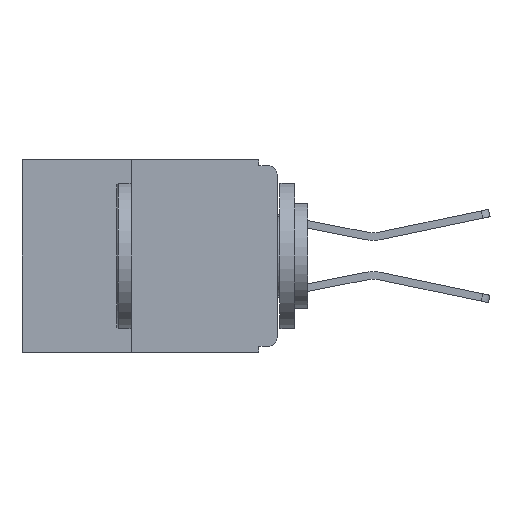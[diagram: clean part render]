
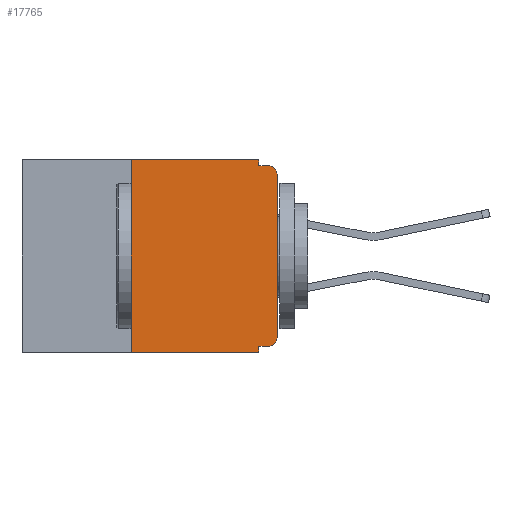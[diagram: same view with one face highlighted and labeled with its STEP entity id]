
A CAD part, left-side view. The second image highlights one B-rep face of the part: STEP entity #17765.
In plain terms, the highlighted planar face has unit normal (-1, 0, 0).
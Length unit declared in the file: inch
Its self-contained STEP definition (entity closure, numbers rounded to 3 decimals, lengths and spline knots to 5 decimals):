
#1190 = EDGE_CURVE ( 'NONE', #27178, #13181, #30315, .T. ) ;
#1698 = CARTESIAN_POINT ( 'NONE',  ( 0., 0.031, -0.32 ) ) ;
#1890 = ORIENTED_EDGE ( 'NONE', *, *, #15229, .T. ) ;
#2044 = CARTESIAN_POINT ( 'NONE',  ( 0., 0., -0.32 ) ) ;
#2105 = VERTEX_POINT ( 'NONE', #14401 ) ;
#2422 = FACE_OUTER_BOUND ( 'NONE', #13908, .T. ) ;
#2535 = EDGE_CURVE ( 'NONE', #2105, #15382, #26771, .T. ) ;
#3551 = DIRECTION ( 'NONE',  ( 0., -1., 0. ) ) ;
#4526 = VERTEX_POINT ( 'NONE', #29566 ) ;
#4619 = CIRCLE ( 'NONE', #5890, 0.015 ) ;
#4720 = DIRECTION ( 'NONE',  ( 0., 0., -1. ) ) ;
#4941 = ORIENTED_EDGE ( 'NONE', *, *, #5636, .F. ) ;
#5055 = EDGE_CURVE ( 'NONE', #17102, #7187, #18247, .T. ) ;
#5384 = CARTESIAN_POINT ( 'NONE',  ( 0., 0.015, -0.025 ) ) ;
#5439 = CARTESIAN_POINT ( 'NONE',  ( 0., 0.437, 0. ) ) ;
#5475 = CARTESIAN_POINT ( 'NONE',  ( 0., 0.031, 0. ) ) ;
#5487 = DIRECTION ( 'NONE',  ( 0., -1., 0. ) ) ;
#5618 = VECTOR ( 'NONE', #21946, 39.37008 ) ;
#5636 = EDGE_CURVE ( 'NONE', #7187, #4526, #25058, .T. ) ;
#5670 = VERTEX_POINT ( 'NONE', #21324 ) ;
#5890 = AXIS2_PLACEMENT_3D ( 'NONE', #5384, #22429, #7809 ) ;
#6074 = ORIENTED_EDGE ( 'NONE', *, *, #1190, .F. ) ;
#7187 = VERTEX_POINT ( 'NONE', #10266 ) ;
#7809 = DIRECTION ( 'NONE',  ( 0., 0., -1. ) ) ;
#8346 = CARTESIAN_POINT ( 'NONE',  ( 0., 0.015, -0.305 ) ) ;
#8969 = CARTESIAN_POINT ( 'NONE',  ( 0., 0.25, 0. ) ) ;
#9055 = CARTESIAN_POINT ( 'NONE',  ( 0., 0., 0. ) ) ;
#9332 = EDGE_CURVE ( 'NONE', #27122, #5670, #20014, .T. ) ;
#10266 = CARTESIAN_POINT ( 'NONE',  ( 0., 0.031, -0.01 ) ) ;
#10271 = CARTESIAN_POINT ( 'NONE',  ( 0., 0.437, -0.33 ) ) ;
#10335 = EDGE_CURVE ( 'NONE', #2105, #13181, #24128, .T. ) ;
#10840 = DIRECTION ( 'NONE',  ( 0., 0., -1. ) ) ;
#11438 = LINE ( 'NONE', #25497, #30891 ) ;
#11677 = VERTEX_POINT ( 'NONE', #17788 ) ;
#11937 = VECTOR ( 'NONE', #5487, 39.37008 ) ;
#12082 = CARTESIAN_POINT ( 'NONE',  ( 0., 0.031, 0. ) ) ;
#12587 = ORIENTED_EDGE ( 'NONE', *, *, #30724, .F. ) ;
#12804 = DIRECTION ( 'NONE',  ( 1., 0., 0. ) ) ;
#13092 = VECTOR ( 'NONE', #27851, 39.37008 ) ;
#13181 = VERTEX_POINT ( 'NONE', #20124 ) ;
#13642 = CARTESIAN_POINT ( 'NONE',  ( 0., 0., -0.305 ) ) ;
#13786 = EDGE_CURVE ( 'NONE', #5670, #4526, #4619, .T. ) ;
#13908 = EDGE_LOOP ( 'NONE', ( #14840, #23605, #4941, #25131, #19818, #14471, #29713, #6074, #12587, #1890 ) ) ;
#13986 = EDGE_CURVE ( 'NONE', #15382, #17102, #11438, .T. ) ;
#14401 = CARTESIAN_POINT ( 'NONE',  ( 0., 0.25, -0.33 ) ) ;
#14471 = ORIENTED_EDGE ( 'NONE', *, *, #2535, .F. ) ;
#14840 = ORIENTED_EDGE ( 'NONE', *, *, #9332, .T. ) ;
#15229 = EDGE_CURVE ( 'NONE', #11677, #27122, #18995, .T. ) ;
#15382 = VERTEX_POINT ( 'NONE', #8969 ) ;
#17102 = VERTEX_POINT ( 'NONE', #12082 ) ;
#17206 = CARTESIAN_POINT ( 'NONE',  ( 0., 0.031, -0.33 ) ) ;
#17574 = AXIS2_PLACEMENT_3D ( 'NONE', #8346, #25427, #10840 ) ;
#17765 = ADVANCED_FACE ( 'NONE', ( #2422 ), #27368, .F. ) ;
#17788 = CARTESIAN_POINT ( 'NONE',  ( 0., 0.015, -0.32 ) ) ;
#18247 = LINE ( 'NONE', #5475, #30434 ) ;
#18971 = DIRECTION ( 'NONE',  ( 0., 0., -1. ) ) ;
#18995 = CIRCLE ( 'NONE', #17574, 0.015 ) ;
#19093 = DIRECTION ( 'NONE',  ( 0., 1., 0. ) ) ;
#19818 = ORIENTED_EDGE ( 'NONE', *, *, #13986, .F. ) ;
#20014 = LINE ( 'NONE', #9055, #26473 ) ;
#20124 = CARTESIAN_POINT ( 'NONE',  ( 0., 0.031, -0.33 ) ) ;
#21324 = CARTESIAN_POINT ( 'NONE',  ( 0., 0., -0.025 ) ) ;
#21946 = DIRECTION ( 'NONE',  ( 0., -1., 0. ) ) ;
#22004 = VECTOR ( 'NONE', #19093, 39.37008 ) ;
#22165 = CARTESIAN_POINT ( 'NONE',  ( 0., 0., -0.01 ) ) ;
#22429 = DIRECTION ( 'NONE',  ( -1., 0., 0. ) ) ;
#23605 = ORIENTED_EDGE ( 'NONE', *, *, #13786, .T. ) ;
#23832 = VECTOR ( 'NONE', #18971, 39.37008 ) ;
#24128 = LINE ( 'NONE', #10271, #11937 ) ;
#25058 = LINE ( 'NONE', #22165, #5618 ) ;
#25131 = ORIENTED_EDGE ( 'NONE', *, *, #5055, .F. ) ;
#25427 = DIRECTION ( 'NONE',  ( -1., 0., 0. ) ) ;
#25497 = CARTESIAN_POINT ( 'NONE',  ( 0., 0.437, 0. ) ) ;
#26182 = LINE ( 'NONE', #2044, #22004 ) ;
#26473 = VECTOR ( 'NONE', #28572, 39.37008 ) ;
#26771 = LINE ( 'NONE', #27401, #13092 ) ;
#27122 = VERTEX_POINT ( 'NONE', #13642 ) ;
#27178 = VERTEX_POINT ( 'NONE', #1698 ) ;
#27368 = PLANE ( 'NONE',  #28853 ) ;
#27401 = CARTESIAN_POINT ( 'NONE',  ( 0., 0.25, -0.33 ) ) ;
#27851 = DIRECTION ( 'NONE',  ( 0., 0., 1. ) ) ;
#28572 = DIRECTION ( 'NONE',  ( 0., 0., 1. ) ) ;
#28853 = AXIS2_PLACEMENT_3D ( 'NONE', #5439, #12804, #29830 ) ;
#29566 = CARTESIAN_POINT ( 'NONE',  ( 0., 0.015, -0.01 ) ) ;
#29713 = ORIENTED_EDGE ( 'NONE', *, *, #10335, .T. ) ;
#29830 = DIRECTION ( 'NONE',  ( 0., 0., -1. ) ) ;
#30315 = LINE ( 'NONE', #17206, #23832 ) ;
#30434 = VECTOR ( 'NONE', #4720, 39.37008 ) ;
#30724 = EDGE_CURVE ( 'NONE', #11677, #27178, #26182, .T. ) ;
#30891 = VECTOR ( 'NONE', #3551, 39.37008 ) ;
